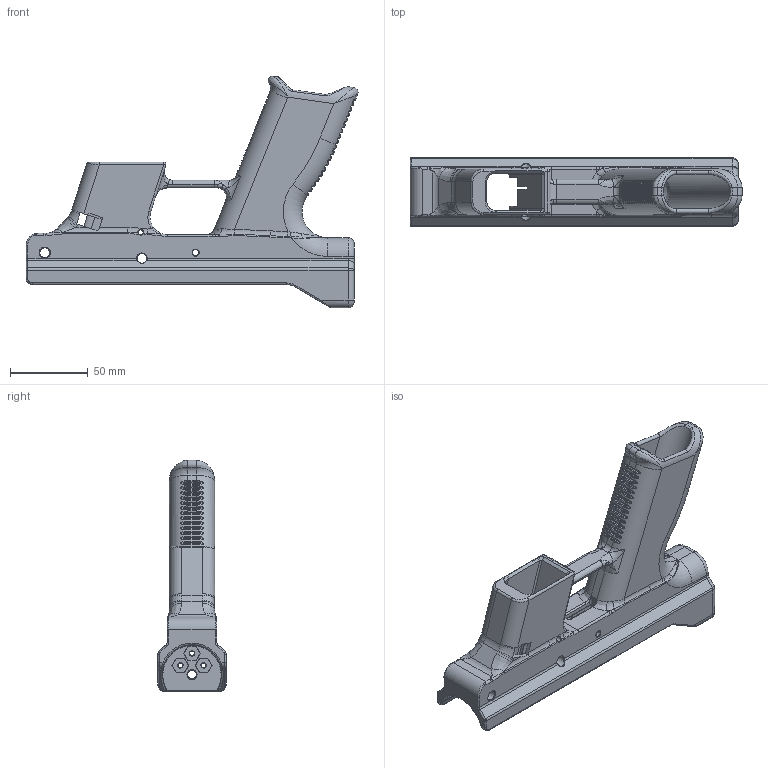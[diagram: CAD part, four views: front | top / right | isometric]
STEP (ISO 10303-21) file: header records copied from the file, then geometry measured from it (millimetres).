
FILE_DESCRIPTION(/* description */ (''),/* implementation_level */ '2;1');
FILE_NAME(/* name */ '513766de-caa5-448f-be74-34fb7392d501.stp',/* time_stamp */ '2019-04-26T13:12:42-04:00',/* author */ (''),/* organization */ (''),/* preprocessor_version */ 'ST-DEVELOPER v18',/* originating_system */ 'Autodesk Translation Framework v8.2.0.1029',/* authorisation */ '');
FILE_SCHEMA (('AUTOMOTIVE_DESIGN { 1 0 10303 214 3 1 1 }'));
Length unit declared in the file: millimetre
Products named in the file (1): FreeMansGhettoBlaster
Bounding box: 213.37 x 44 x 148.84 mm (x, y, z)
Volume: 225112.7 mm3; surface area: 80597.9 mm2
Topology: 1 solids, 1 shells, 980 faces, 2386 edges, 1369 vertices
Faces by surface type: bspline 387, cylinder 272, plane 222, torus 72, cone 25, sphere 2
Full cylindrical faces by diameter (mm): 3 x3, 3.175 x2, 4 x2, 5.5 x1, 6.3 x4
Entity records: 41414 total; most frequent: CARTESIAN_POINT 20204, ORIENTED_EDGE 4718, DIRECTION 4003, EDGE_CURVE 2359, AXIS2_PLACEMENT_3D 1596, VERTEX_POINT 1370, EDGE_LOOP 1003, FACE_OUTER_BOUND 980
